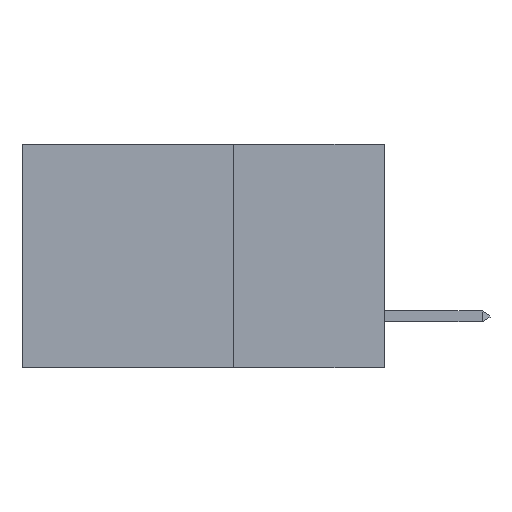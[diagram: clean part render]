
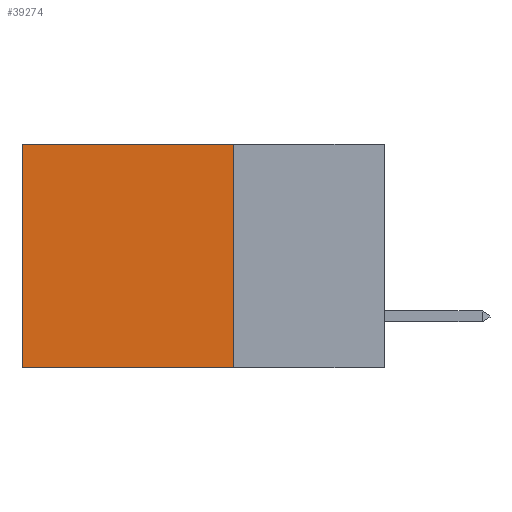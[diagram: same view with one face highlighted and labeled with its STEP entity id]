
A CAD part, left-side view. The second image highlights one B-rep face of the part: STEP entity #39274.
In plain terms, the highlighted planar face has unit normal (-1, 0, 0).
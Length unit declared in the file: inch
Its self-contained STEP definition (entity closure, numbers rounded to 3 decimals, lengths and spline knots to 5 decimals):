
#66 = VERTEX_POINT ( 'NONE', #17221 ) ;
#393 = ORIENTED_EDGE ( 'NONE', *, *, #25014, .T. ) ;
#726 = EDGE_CURVE ( 'NONE', #16823, #1312, #13370, .T. ) ;
#1119 = DIRECTION ( 'NONE',  ( 1., 0., 0. ) ) ;
#1312 = VERTEX_POINT ( 'NONE', #39492 ) ;
#2430 = DIRECTION ( 'NONE',  ( 0., 1., 0. ) ) ;
#3672 = ORIENTED_EDGE ( 'NONE', *, *, #18793, .F. ) ;
#4875 = CARTESIAN_POINT ( 'NONE',  ( 0.2875, 0.25, -0.37 ) ) ;
#4962 = DIRECTION ( 'NONE',  ( 0., 0., -1. ) ) ;
#6669 = FACE_OUTER_BOUND ( 'NONE', #18055, .T. ) ;
#9293 = LINE ( 'NONE', #34332, #25268 ) ;
#9468 = VERTEX_POINT ( 'NONE', #40736 ) ;
#13370 = LINE ( 'NONE', #27082, #37690 ) ;
#13687 = PLANE ( 'NONE',  #30561 ) ;
#14420 = DIRECTION ( 'NONE',  ( 0., 1., 0. ) ) ;
#16823 = VERTEX_POINT ( 'NONE', #29442 ) ;
#17221 = CARTESIAN_POINT ( 'NONE',  ( 0.2875, 0.25, -0.37 ) ) ;
#17261 = VECTOR ( 'NONE', #2430, 39.37008 ) ;
#18055 = EDGE_LOOP ( 'NONE', ( #22051, #3672, #37822, #393 ) ) ;
#18279 = LINE ( 'NONE', #21493, #17261 ) ;
#18793 = EDGE_CURVE ( 'NONE', #66, #1312, #28446, .T. ) ;
#20167 = CARTESIAN_POINT ( 'NONE',  ( 0.2875, 0.25, 0. ) ) ;
#21493 = CARTESIAN_POINT ( 'NONE',  ( 0.2875, 0.25, 0. ) ) ;
#22051 = ORIENTED_EDGE ( 'NONE', *, *, #726, .T. ) ;
#23403 = DIRECTION ( 'NONE',  ( 0., 0., -1. ) ) ;
#25014 = EDGE_CURVE ( 'NONE', #9468, #16823, #18279, .T. ) ;
#25268 = VECTOR ( 'NONE', #40551, 39.37008 ) ;
#27082 = CARTESIAN_POINT ( 'NONE',  ( 0.2875, 0.6, 0. ) ) ;
#27494 = VECTOR ( 'NONE', #14420, 39.37008 ) ;
#28446 = LINE ( 'NONE', #4875, #27494 ) ;
#29442 = CARTESIAN_POINT ( 'NONE',  ( 0.2875, 0.6, 0. ) ) ;
#30561 = AXIS2_PLACEMENT_3D ( 'NONE', #20167, #1119, #23403 ) ;
#34332 = CARTESIAN_POINT ( 'NONE',  ( 0.2875, 0.25, 0. ) ) ;
#35356 = EDGE_CURVE ( 'NONE', #9468, #66, #9293, .T. ) ;
#37690 = VECTOR ( 'NONE', #4962, 39.37008 ) ;
#37822 = ORIENTED_EDGE ( 'NONE', *, *, #35356, .F. ) ;
#39274 = ADVANCED_FACE ( 'NONE', ( #6669 ), #13687, .F. ) ;
#39492 = CARTESIAN_POINT ( 'NONE',  ( 0.2875, 0.6, -0.37 ) ) ;
#40551 = DIRECTION ( 'NONE',  ( 0., 0., -1. ) ) ;
#40736 = CARTESIAN_POINT ( 'NONE',  ( 0.2875, 0.25, 0. ) ) ;
